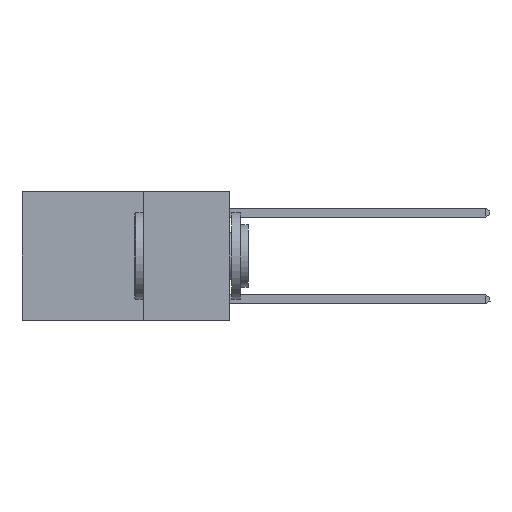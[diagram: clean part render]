
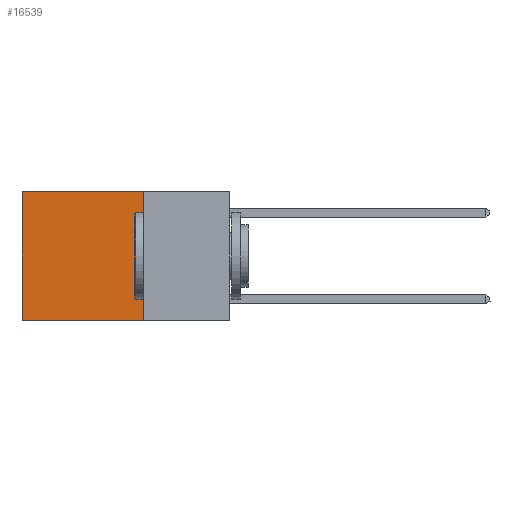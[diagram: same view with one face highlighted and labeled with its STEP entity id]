
A CAD part, left-side view. The second image highlights one B-rep face of the part: STEP entity #16539.
In plain terms, the highlighted planar face has unit normal (-1, 0, 0).
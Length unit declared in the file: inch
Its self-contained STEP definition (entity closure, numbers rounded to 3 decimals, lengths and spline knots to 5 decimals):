
#1295 = ORIENTED_EDGE ( 'NONE', *, *, #7215, .F. ) ;
#1497 = VERTEX_POINT ( 'NONE', #9583 ) ;
#1523 = DIRECTION ( 'NONE',  ( 0., 0., -1. ) ) ;
#1692 = LINE ( 'NONE', #10204, #6077 ) ;
#2825 = LINE ( 'NONE', #5773, #13312 ) ;
#3052 = PLANE ( 'NONE',  #17399 ) ;
#3786 = DIRECTION ( 'NONE',  ( 0., 1., 0. ) ) ;
#5773 = CARTESIAN_POINT ( 'NONE',  ( 0.2625, 0.6, 0. ) ) ;
#6077 = VECTOR ( 'NONE', #1523, 39.37008 ) ;
#7011 = EDGE_CURVE ( 'NONE', #14447, #1497, #17975, .T. ) ;
#7184 = EDGE_CURVE ( 'NONE', #12072, #1497, #2825, .T. ) ;
#7215 = EDGE_CURVE ( 'NONE', #16059, #14447, #1692, .T. ) ;
#8821 = CARTESIAN_POINT ( 'NONE',  ( 0.2625, 0.25, 0. ) ) ;
#9296 = EDGE_CURVE ( 'NONE', #16059, #12072, #11433, .T. ) ;
#9583 = CARTESIAN_POINT ( 'NONE',  ( 0.2625, 0.6, -0.37 ) ) ;
#9898 = VECTOR ( 'NONE', #16444, 39.37008 ) ;
#10204 = CARTESIAN_POINT ( 'NONE',  ( 0.2625, 0.25, 0. ) ) ;
#10235 = FACE_OUTER_BOUND ( 'NONE', #10986, .T. ) ;
#10319 = DIRECTION ( 'NONE',  ( 0., 0., -1. ) ) ;
#10673 = CARTESIAN_POINT ( 'NONE',  ( 0.2625, 0.25, -0.37 ) ) ;
#10986 = EDGE_LOOP ( 'NONE', ( #15517, #12181, #1295, #11948 ) ) ;
#11433 = LINE ( 'NONE', #15311, #14609 ) ;
#11948 = ORIENTED_EDGE ( 'NONE', *, *, #9296, .T. ) ;
#12072 = VERTEX_POINT ( 'NONE', #17796 ) ;
#12181 = ORIENTED_EDGE ( 'NONE', *, *, #7011, .F. ) ;
#13312 = VECTOR ( 'NONE', #17508, 39.37008 ) ;
#13736 = CARTESIAN_POINT ( 'NONE',  ( 0.2625, 0.25, -0.37 ) ) ;
#14447 = VERTEX_POINT ( 'NONE', #13736 ) ;
#14565 = DIRECTION ( 'NONE',  ( 1., 0., 0. ) ) ;
#14609 = VECTOR ( 'NONE', #3786, 39.37008 ) ;
#15311 = CARTESIAN_POINT ( 'NONE',  ( 0.2625, 0.25, 0. ) ) ;
#15517 = ORIENTED_EDGE ( 'NONE', *, *, #7184, .T. ) ;
#16059 = VERTEX_POINT ( 'NONE', #16586 ) ;
#16444 = DIRECTION ( 'NONE',  ( 0., 1., 0. ) ) ;
#16539 = ADVANCED_FACE ( 'NONE', ( #10235 ), #3052, .F. ) ;
#16586 = CARTESIAN_POINT ( 'NONE',  ( 0.2625, 0.25, 0. ) ) ;
#17399 = AXIS2_PLACEMENT_3D ( 'NONE', #8821, #14565, #10319 ) ;
#17508 = DIRECTION ( 'NONE',  ( 0., 0., -1. ) ) ;
#17796 = CARTESIAN_POINT ( 'NONE',  ( 0.2625, 0.6, 0. ) ) ;
#17975 = LINE ( 'NONE', #10673, #9898 ) ;
